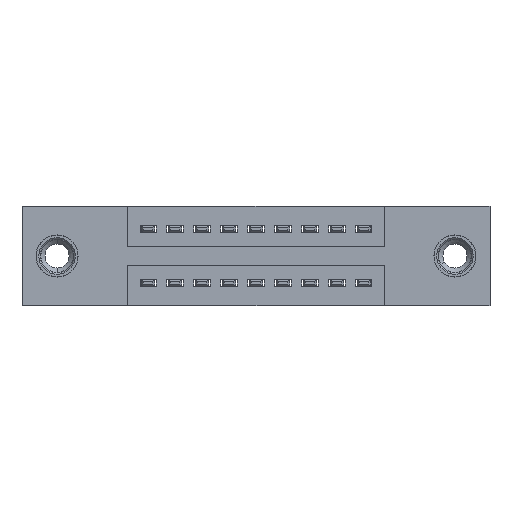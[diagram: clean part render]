
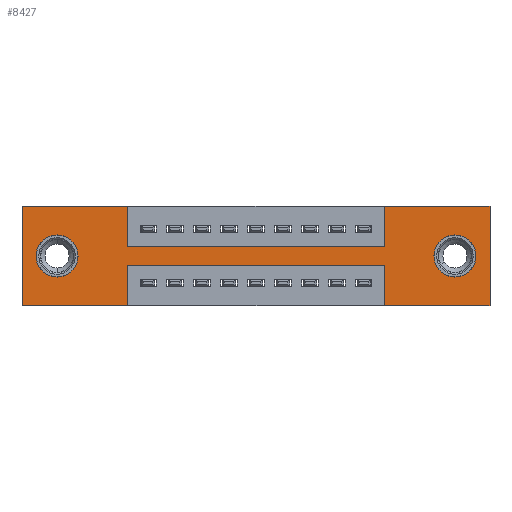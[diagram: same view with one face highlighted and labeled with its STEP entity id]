
A CAD part, front view. The second image highlights one B-rep face of the part: STEP entity #8427.
In plain terms, the highlighted planar face has unit normal (0, -1, 0).
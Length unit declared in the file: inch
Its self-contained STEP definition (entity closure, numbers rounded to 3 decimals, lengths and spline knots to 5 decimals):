
#92 = DIRECTION ( 'NONE',  ( 0., 0., 1. ) ) ;
#112 = DIRECTION ( 'NONE',  ( 0., 0., 1. ) ) ;
#122 = LINE ( 'NONE', #4772, #7525 ) ;
#277 = AXIS2_PLACEMENT_3D ( 'NONE', #4726, #6677, #5678 ) ;
#352 = DIRECTION ( 'NONE',  ( -1., 0., 0. ) ) ;
#360 = CARTESIAN_POINT ( 'NONE',  ( 0., 0., -0.37 ) ) ;
#467 = LINE ( 'NONE', #8913, #6645 ) ;
#485 = VERTEX_POINT ( 'NONE', #7804 ) ;
#617 = AXIS2_PLACEMENT_3D ( 'NONE', #8192, #2513, #12210 ) ;
#680 = ORIENTED_EDGE ( 'NONE', *, *, #9600, .F. ) ;
#688 = VECTOR ( 'NONE', #8654, 39.37008 ) ;
#794 = AXIS2_PLACEMENT_3D ( 'NONE', #2625, #6473, #6594 ) ;
#1008 = CARTESIAN_POINT ( 'NONE',  ( 1.3425, 0., -0.22 ) ) ;
#1088 = ORIENTED_EDGE ( 'NONE', *, *, #2069, .F. ) ;
#1106 = EDGE_CURVE ( 'NONE', #10105, #2348, #12080, .T. ) ;
#1209 = CIRCLE ( 'NONE', #617, 0.078 ) ;
#1294 = VERTEX_POINT ( 'NONE', #12223 ) ;
#1295 = EDGE_CURVE ( 'NONE', #6681, #3298, #6469, .T. ) ;
#1468 = DIRECTION ( 'NONE',  ( 1., 0., 0. ) ) ;
#1483 = VECTOR ( 'NONE', #112, 39.37008 ) ;
#1505 = LINE ( 'NONE', #9049, #10590 ) ;
#1524 = FACE_OUTER_BOUND ( 'NONE', #7009, .T. ) ;
#1697 = EDGE_CURVE ( 'NONE', #3298, #7127, #122, .T. ) ;
#1706 = CARTESIAN_POINT ( 'NONE',  ( 1.605, 0., -0.263 ) ) ;
#1806 = DIRECTION ( 'NONE',  ( 0., 0., -1. ) ) ;
#2069 = EDGE_CURVE ( 'NONE', #7954, #3828, #5233, .T. ) ;
#2226 = ORIENTED_EDGE ( 'NONE', *, *, #1295, .F. ) ;
#2239 = VERTEX_POINT ( 'NONE', #1706 ) ;
#2348 = VERTEX_POINT ( 'NONE', #3602 ) ;
#2513 = DIRECTION ( 'NONE',  ( 0., 1., 0. ) ) ;
#2624 = ORIENTED_EDGE ( 'NONE', *, *, #9549, .F. ) ;
#2625 = CARTESIAN_POINT ( 'NONE',  ( 0.13, 0., -0.185 ) ) ;
#2706 = DIRECTION ( 'NONE',  ( 1., 0., 0. ) ) ;
#2799 = EDGE_CURVE ( 'NONE', #10410, #9931, #10973, .T. ) ;
#2956 = CARTESIAN_POINT ( 'NONE',  ( 0., 0., 0. ) ) ;
#3035 = EDGE_LOOP ( 'NONE', ( #4732, #9154 ) ) ;
#3073 = CARTESIAN_POINT ( 'NONE',  ( 0., 0., 0. ) ) ;
#3151 = DIRECTION ( 'NONE',  ( -1., 0., 0. ) ) ;
#3177 = FACE_BOUND ( 'NONE', #3035, .T. ) ;
#3223 = ORIENTED_EDGE ( 'NONE', *, *, #6825, .T. ) ;
#3298 = VERTEX_POINT ( 'NONE', #12171 ) ;
#3336 = DIRECTION ( 'NONE',  ( 0., 0., 1. ) ) ;
#3602 = CARTESIAN_POINT ( 'NONE',  ( 0.13, 0., -0.107 ) ) ;
#3828 = VERTEX_POINT ( 'NONE', #7794 ) ;
#3929 = CARTESIAN_POINT ( 'NONE',  ( 0.3925, 0., -0.15 ) ) ;
#4003 = CARTESIAN_POINT ( 'NONE',  ( 0.3925, 0., -0.22 ) ) ;
#4029 = ORIENTED_EDGE ( 'NONE', *, *, #8533, .F. ) ;
#4266 = AXIS2_PLACEMENT_3D ( 'NONE', #5141, #9974, #6117 ) ;
#4425 = ORIENTED_EDGE ( 'NONE', *, *, #6575, .F. ) ;
#4543 = CARTESIAN_POINT ( 'NONE',  ( 0., 0., -0.37 ) ) ;
#4726 = CARTESIAN_POINT ( 'NONE',  ( 0., 0., -0.37 ) ) ;
#4732 = ORIENTED_EDGE ( 'NONE', *, *, #10719, .T. ) ;
#4772 = CARTESIAN_POINT ( 'NONE',  ( 1.3425, 0., 0. ) ) ;
#4802 = CIRCLE ( 'NONE', #4266, 0.078 ) ;
#4954 = CARTESIAN_POINT ( 'NONE',  ( 0.3925, 0., -0.22 ) ) ;
#4983 = CARTESIAN_POINT ( 'NONE',  ( 0.13, 0., -0.263 ) ) ;
#5141 = CARTESIAN_POINT ( 'NONE',  ( 1.605, 0., -0.185 ) ) ;
#5153 = FACE_BOUND ( 'NONE', #9143, .T. ) ;
#5207 = VECTOR ( 'NONE', #8976, 39.37008 ) ;
#5233 = LINE ( 'NONE', #3073, #9774 ) ;
#5447 = VECTOR ( 'NONE', #92, 39.37008 ) ;
#5601 = ORIENTED_EDGE ( 'NONE', *, *, #9680, .F. ) ;
#5678 = DIRECTION ( 'NONE',  ( 0., 0., -1. ) ) ;
#5724 = LINE ( 'NONE', #4003, #7706 ) ;
#6117 = DIRECTION ( 'NONE',  ( 0., 0., -1. ) ) ;
#6428 = CARTESIAN_POINT ( 'NONE',  ( 0.3925, 0., -0.37 ) ) ;
#6437 = DIRECTION ( 'NONE',  ( 0., 1., 0. ) ) ;
#6469 = LINE ( 'NONE', #11970, #8895 ) ;
#6473 = DIRECTION ( 'NONE',  ( 0., 1., 0. ) ) ;
#6575 = EDGE_CURVE ( 'NONE', #3828, #6681, #11873, .T. ) ;
#6594 = DIRECTION ( 'NONE',  ( 0., 0., 1. ) ) ;
#6645 = VECTOR ( 'NONE', #7928, 39.37008 ) ;
#6677 = DIRECTION ( 'NONE',  ( 0., -1., 0. ) ) ;
#6681 = VERTEX_POINT ( 'NONE', #3929 ) ;
#6825 = EDGE_CURVE ( 'NONE', #2348, #10105, #9447, .T. ) ;
#6845 = ORIENTED_EDGE ( 'NONE', *, *, #7619, .F. ) ;
#7001 = VECTOR ( 'NONE', #2706, 39.37008 ) ;
#7009 = EDGE_LOOP ( 'NONE', ( #5601, #2624, #4029, #680, #6845, #10614, #11405, #2226, #4425, #1088, #10452, #7509 ) ) ;
#7081 = CARTESIAN_POINT ( 'NONE',  ( 0., 0., 0. ) ) ;
#7127 = VERTEX_POINT ( 'NONE', #11507 ) ;
#7277 = VERTEX_POINT ( 'NONE', #4954 ) ;
#7509 = ORIENTED_EDGE ( 'NONE', *, *, #2799, .F. ) ;
#7525 = VECTOR ( 'NONE', #11701, 39.37008 ) ;
#7531 = CARTESIAN_POINT ( 'NONE',  ( 1.735, 0., 0. ) ) ;
#7555 = CARTESIAN_POINT ( 'NONE',  ( 1.735, 0., -0.37 ) ) ;
#7619 = EDGE_CURVE ( 'NONE', #1294, #8879, #12454, .T. ) ;
#7661 = CARTESIAN_POINT ( 'NONE',  ( 0., 0., 0. ) ) ;
#7706 = VECTOR ( 'NONE', #352, 39.37008 ) ;
#7759 = VERTEX_POINT ( 'NONE', #1008 ) ;
#7794 = CARTESIAN_POINT ( 'NONE',  ( 0.3925, 0., 0. ) ) ;
#7804 = CARTESIAN_POINT ( 'NONE',  ( 1.605, 0., -0.107 ) ) ;
#7928 = DIRECTION ( 'NONE',  ( 0., 0., -1. ) ) ;
#7954 = VERTEX_POINT ( 'NONE', #7081 ) ;
#8153 = VERTEX_POINT ( 'NONE', #11224 ) ;
#8192 = CARTESIAN_POINT ( 'NONE',  ( 1.605, 0., -0.185 ) ) ;
#8252 = EDGE_CURVE ( 'NONE', #7127, #1294, #8503, .T. ) ;
#8427 = ADVANCED_FACE ( 'NONE', ( #3177, #5153, #1524 ), #9630, .T. ) ;
#8503 = LINE ( 'NONE', #7661, #7001 ) ;
#8533 = EDGE_CURVE ( 'NONE', #8153, #7759, #10005, .T. ) ;
#8651 = ORIENTED_EDGE ( 'NONE', *, *, #1106, .T. ) ;
#8654 = DIRECTION ( 'NONE',  ( 0., 0., -1. ) ) ;
#8684 = EDGE_CURVE ( 'NONE', #2239, #485, #1209, .T. ) ;
#8735 = CARTESIAN_POINT ( 'NONE',  ( 0.3925, 0., 0. ) ) ;
#8879 = VERTEX_POINT ( 'NONE', #7555 ) ;
#8895 = VECTOR ( 'NONE', #1468, 39.37008 ) ;
#8913 = CARTESIAN_POINT ( 'NONE',  ( 0.3925, 0., -0.37 ) ) ;
#8976 = DIRECTION ( 'NONE',  ( -1., 0., 0. ) ) ;
#9049 = CARTESIAN_POINT ( 'NONE',  ( 0., 0., -0.37 ) ) ;
#9129 = VECTOR ( 'NONE', #1806, 39.37008 ) ;
#9143 = EDGE_LOOP ( 'NONE', ( #3223, #8651 ) ) ;
#9154 = ORIENTED_EDGE ( 'NONE', *, *, #8684, .T. ) ;
#9331 = CARTESIAN_POINT ( 'NONE',  ( 0.13, 0., -0.185 ) ) ;
#9447 = CIRCLE ( 'NONE', #10720, 0.078 ) ;
#9549 = EDGE_CURVE ( 'NONE', #7759, #7277, #5724, .T. ) ;
#9600 = EDGE_CURVE ( 'NONE', #8879, #8153, #1505, .T. ) ;
#9630 = PLANE ( 'NONE',  #277 ) ;
#9680 = EDGE_CURVE ( 'NONE', #7277, #10410, #467, .T. ) ;
#9774 = VECTOR ( 'NONE', #9899, 39.37008 ) ;
#9796 = CARTESIAN_POINT ( 'NONE',  ( 1.3425, 0., -0.37 ) ) ;
#9899 = DIRECTION ( 'NONE',  ( 1., 0., 0. ) ) ;
#9931 = VERTEX_POINT ( 'NONE', #4543 ) ;
#9974 = DIRECTION ( 'NONE',  ( 0., 1., 0. ) ) ;
#10005 = LINE ( 'NONE', #9796, #5447 ) ;
#10105 = VERTEX_POINT ( 'NONE', #4983 ) ;
#10201 = EDGE_CURVE ( 'NONE', #9931, #7954, #11037, .T. ) ;
#10410 = VERTEX_POINT ( 'NONE', #6428 ) ;
#10452 = ORIENTED_EDGE ( 'NONE', *, *, #10201, .F. ) ;
#10590 = VECTOR ( 'NONE', #3151, 39.37008 ) ;
#10614 = ORIENTED_EDGE ( 'NONE', *, *, #8252, .F. ) ;
#10719 = EDGE_CURVE ( 'NONE', #485, #2239, #4802, .T. ) ;
#10720 = AXIS2_PLACEMENT_3D ( 'NONE', #9331, #6437, #3336 ) ;
#10973 = LINE ( 'NONE', #360, #5207 ) ;
#11037 = LINE ( 'NONE', #2956, #1483 ) ;
#11224 = CARTESIAN_POINT ( 'NONE',  ( 1.3425, 0., -0.37 ) ) ;
#11405 = ORIENTED_EDGE ( 'NONE', *, *, #1697, .F. ) ;
#11507 = CARTESIAN_POINT ( 'NONE',  ( 1.3425, 0., 0. ) ) ;
#11701 = DIRECTION ( 'NONE',  ( 0., 0., 1. ) ) ;
#11873 = LINE ( 'NONE', #8735, #688 ) ;
#11970 = CARTESIAN_POINT ( 'NONE',  ( 0.3925, 0., -0.15 ) ) ;
#12080 = CIRCLE ( 'NONE', #794, 0.078 ) ;
#12171 = CARTESIAN_POINT ( 'NONE',  ( 1.3425, 0., -0.15 ) ) ;
#12210 = DIRECTION ( 'NONE',  ( 0., 0., -1. ) ) ;
#12223 = CARTESIAN_POINT ( 'NONE',  ( 1.735, 0., 0. ) ) ;
#12454 = LINE ( 'NONE', #7531, #9129 ) ;
